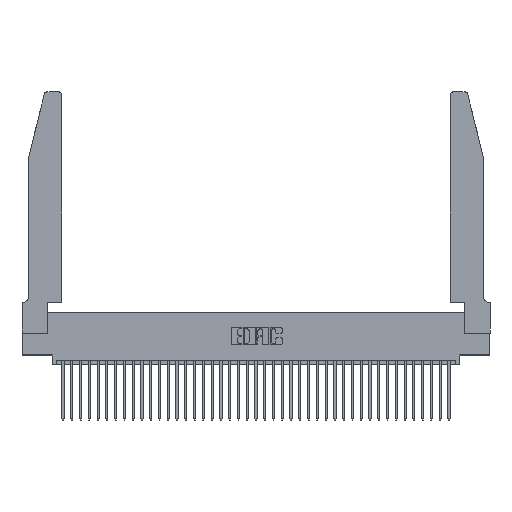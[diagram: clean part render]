
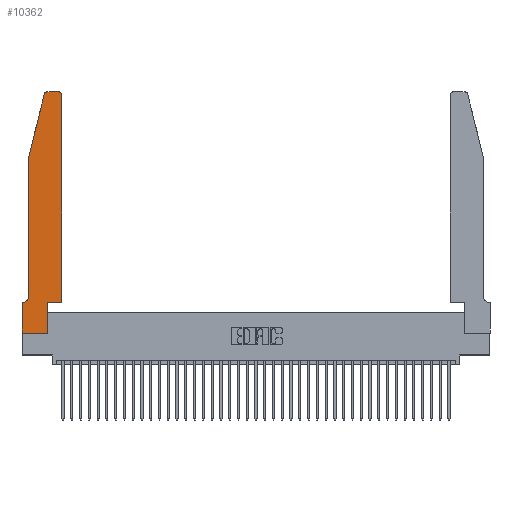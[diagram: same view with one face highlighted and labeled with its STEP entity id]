
A CAD part, top view. The second image highlights one B-rep face of the part: STEP entity #10362.
In plain terms, the highlighted planar face has unit normal (0, 0, 1).
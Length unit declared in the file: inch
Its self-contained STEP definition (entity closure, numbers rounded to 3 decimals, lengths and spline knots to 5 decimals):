
#124 = CIRCLE ( 'NONE', #20046, 0.03 ) ;
#319 = CARTESIAN_POINT ( 'NONE',  ( 0.4205, 2.72, 0.37 ) ) ;
#351 = PLANE ( 'NONE',  #27690 ) ;
#1141 = DIRECTION ( 'NONE',  ( 0., 1., 0. ) ) ;
#1270 = CARTESIAN_POINT ( 'NONE',  ( 0.0755, 0.35, 0.37 ) ) ;
#2204 = CARTESIAN_POINT ( 'NONE',  ( 0.0755, 2., 0.37 ) ) ;
#2300 = CARTESIAN_POINT ( 'NONE',  ( 0.284, 2.75, 0.37 ) ) ;
#2797 = VERTEX_POINT ( 'NONE', #2300 ) ;
#3397 = EDGE_CURVE ( 'NONE', #38675, #5653, #12107, .T. ) ;
#3466 = DIRECTION ( 'NONE',  ( 1., 0., 0. ) ) ;
#3772 = VECTOR ( 'NONE', #30601, 39.37008 ) ;
#3882 = EDGE_CURVE ( 'NONE', #7929, #23700, #28379, .T. ) ;
#4121 = DIRECTION ( 'NONE',  ( 0., 1., 0. ) ) ;
#4732 = EDGE_CURVE ( 'NONE', #24417, #7929, #22162, .T. ) ;
#4800 = CARTESIAN_POINT ( 'NONE',  ( 0.4505, 0.35, 0.37 ) ) ;
#5131 = AXIS2_PLACEMENT_3D ( 'NONE', #36051, #17753, #39092 ) ;
#5587 = EDGE_LOOP ( 'NONE', ( #38892, #19785, #23565, #16771, #8505, #27211, #10316, #10397, #20698, #25689, #9909, #33874 ) ) ;
#5653 = VERTEX_POINT ( 'NONE', #9464 ) ;
#5666 = DIRECTION ( 'NONE',  ( -0.239, -0.971, 0. ) ) ;
#5716 = VECTOR ( 'NONE', #26966, 39.37008 ) ;
#6600 = LINE ( 'NONE', #12273, #21090 ) ;
#7665 = EDGE_CURVE ( 'NONE', #5653, #24098, #36445, .T. ) ;
#7823 = CARTESIAN_POINT ( 'NONE',  ( 0.4205, 2.75, 0.37 ) ) ;
#7850 = LINE ( 'NONE', #37787, #23263 ) ;
#7927 = DIRECTION ( 'NONE',  ( 1., 0., 0. ) ) ;
#7929 = VERTEX_POINT ( 'NONE', #37754 ) ;
#8187 = VECTOR ( 'NONE', #7927, 39.37008 ) ;
#8293 = DIRECTION ( 'NONE',  ( 0., 0., -1. ) ) ;
#8505 = ORIENTED_EDGE ( 'NONE', *, *, #3397, .T. ) ;
#9062 = EDGE_CURVE ( 'NONE', #39755, #2797, #6600, .T. ) ;
#9390 = VERTEX_POINT ( 'NONE', #32063 ) ;
#9464 = CARTESIAN_POINT ( 'NONE',  ( 0.0055, 0.35, 0.37 ) ) ;
#9757 = CARTESIAN_POINT ( 'NONE',  ( 0., 0.35, 0.37 ) ) ;
#9909 = ORIENTED_EDGE ( 'NONE', *, *, #23473, .T. ) ;
#10316 = ORIENTED_EDGE ( 'NONE', *, *, #25820, .T. ) ;
#10362 = ADVANCED_FACE ( 'NONE', ( #22506 ), #351, .T. ) ;
#10397 = ORIENTED_EDGE ( 'NONE', *, *, #4732, .T. ) ;
#11014 = EDGE_CURVE ( 'NONE', #9390, #39755, #124, .T. ) ;
#11146 = VECTOR ( 'NONE', #23760, 39.37008 ) ;
#11286 = CARTESIAN_POINT ( 'NONE',  ( 0.2865, 0.35, 0.37 ) ) ;
#11364 = CARTESIAN_POINT ( 'NONE',  ( 0.0755, 2., 0.37 ) ) ;
#12027 = VECTOR ( 'NONE', #29037, 39.37008 ) ;
#12107 = CIRCLE ( 'NONE', #13436, 0.07 ) ;
#12273 = CARTESIAN_POINT ( 'NONE',  ( 0.2605, 2.75, 0.37 ) ) ;
#12852 = DIRECTION ( 'NONE',  ( 1., 0., 0. ) ) ;
#12917 = CARTESIAN_POINT ( 'NONE',  ( 0.4505, 0.35, 0.37 ) ) ;
#13436 = AXIS2_PLACEMENT_3D ( 'NONE', #26674, #8293, #29759 ) ;
#15838 = EDGE_CURVE ( 'NONE', #2797, #39210, #38562, .T. ) ;
#16594 = CARTESIAN_POINT ( 'NONE',  ( 0.2865, 0.35, 0.37 ) ) ;
#16771 = ORIENTED_EDGE ( 'NONE', *, *, #18515, .T. ) ;
#17559 = VERTEX_POINT ( 'NONE', #12917 ) ;
#17753 = DIRECTION ( 'NONE',  ( 0., 0., 1. ) ) ;
#17941 = CARTESIAN_POINT ( 'NONE',  ( 0.0755, 2., 0.37 ) ) ;
#18474 = DIRECTION ( 'NONE',  ( -1., 0., 0. ) ) ;
#18515 = EDGE_CURVE ( 'NONE', #27785, #38675, #25576, .T. ) ;
#18533 = LINE ( 'NONE', #17941, #21915 ) ;
#19522 = EDGE_CURVE ( 'NONE', #23700, #17559, #29789, .T. ) ;
#19785 = ORIENTED_EDGE ( 'NONE', *, *, #15838, .T. ) ;
#20046 = AXIS2_PLACEMENT_3D ( 'NONE', #319, #22019, #3466 ) ;
#20240 = LINE ( 'NONE', #25982, #12027 ) ;
#20698 = ORIENTED_EDGE ( 'NONE', *, *, #3882, .T. ) ;
#20795 = CARTESIAN_POINT ( 'NONE',  ( 0.25487, 2.72718, 0.37 ) ) ;
#20843 = CARTESIAN_POINT ( 'NONE',  ( 0., 0., 0.37 ) ) ;
#20961 = CARTESIAN_POINT ( 'NONE',  ( 0.0755, 0.42, 0.37 ) ) ;
#21090 = VECTOR ( 'NONE', #18474, 39.37008 ) ;
#21915 = VECTOR ( 'NONE', #5666, 39.37008 ) ;
#22019 = DIRECTION ( 'NONE',  ( 0., 0., 1. ) ) ;
#22162 = LINE ( 'NONE', #20843, #5716 ) ;
#22506 = FACE_OUTER_BOUND ( 'NONE', #5587, .T. ) ;
#23263 = VECTOR ( 'NONE', #4121, 39.37008 ) ;
#23473 = EDGE_CURVE ( 'NONE', #17559, #9390, #7850, .T. ) ;
#23565 = ORIENTED_EDGE ( 'NONE', *, *, #36571, .T. ) ;
#23700 = VERTEX_POINT ( 'NONE', #11286 ) ;
#23760 = DIRECTION ( 'NONE',  ( 0., -1., 0. ) ) ;
#24098 = VERTEX_POINT ( 'NONE', #37741 ) ;
#24417 = VERTEX_POINT ( 'NONE', #29896 ) ;
#25576 = LINE ( 'NONE', #11364, #11146 ) ;
#25689 = ORIENTED_EDGE ( 'NONE', *, *, #19522, .T. ) ;
#25820 = EDGE_CURVE ( 'NONE', #24098, #24417, #20240, .T. ) ;
#25982 = CARTESIAN_POINT ( 'NONE',  ( 0., 0., 0.37 ) ) ;
#26674 = CARTESIAN_POINT ( 'NONE',  ( 0.0055, 0.42, 0.37 ) ) ;
#26966 = DIRECTION ( 'NONE',  ( 1., 0., 0. ) ) ;
#27211 = ORIENTED_EDGE ( 'NONE', *, *, #7665, .T. ) ;
#27690 = AXIS2_PLACEMENT_3D ( 'NONE', #9757, #31201, #12852 ) ;
#27785 = VERTEX_POINT ( 'NONE', #2204 ) ;
#28379 = LINE ( 'NONE', #16594, #35539 ) ;
#29037 = DIRECTION ( 'NONE',  ( 0., -1., 0. ) ) ;
#29759 = DIRECTION ( 'NONE',  ( -1., 0., 0. ) ) ;
#29789 = LINE ( 'NONE', #4800, #8187 ) ;
#29896 = CARTESIAN_POINT ( 'NONE',  ( 0., 0., 0.37 ) ) ;
#30601 = DIRECTION ( 'NONE',  ( -1., 0., 0. ) ) ;
#31201 = DIRECTION ( 'NONE',  ( 0., 0., 1. ) ) ;
#32063 = CARTESIAN_POINT ( 'NONE',  ( 0.4505, 2.72, 0.37 ) ) ;
#33874 = ORIENTED_EDGE ( 'NONE', *, *, #11014, .T. ) ;
#35539 = VECTOR ( 'NONE', #1141, 39.37008 ) ;
#36051 = CARTESIAN_POINT ( 'NONE',  ( 0.284, 2.72, 0.37 ) ) ;
#36445 = LINE ( 'NONE', #1270, #3772 ) ;
#36571 = EDGE_CURVE ( 'NONE', #39210, #27785, #18533, .T. ) ;
#37741 = CARTESIAN_POINT ( 'NONE',  ( 0., 0.35, 0.37 ) ) ;
#37754 = CARTESIAN_POINT ( 'NONE',  ( 0.2865, 0., 0.37 ) ) ;
#37787 = CARTESIAN_POINT ( 'NONE',  ( 0.4505, 0.35, 0.37 ) ) ;
#38562 = CIRCLE ( 'NONE', #5131, 0.03 ) ;
#38675 = VERTEX_POINT ( 'NONE', #20961 ) ;
#38892 = ORIENTED_EDGE ( 'NONE', *, *, #9062, .T. ) ;
#39092 = DIRECTION ( 'NONE',  ( 1., 0., 0. ) ) ;
#39210 = VERTEX_POINT ( 'NONE', #20795 ) ;
#39755 = VERTEX_POINT ( 'NONE', #7823 ) ;
